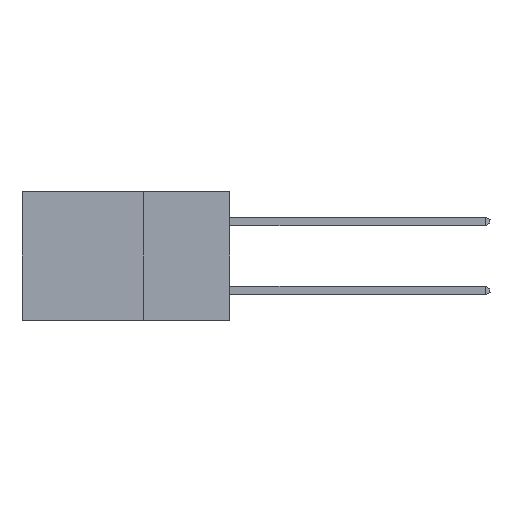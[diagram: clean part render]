
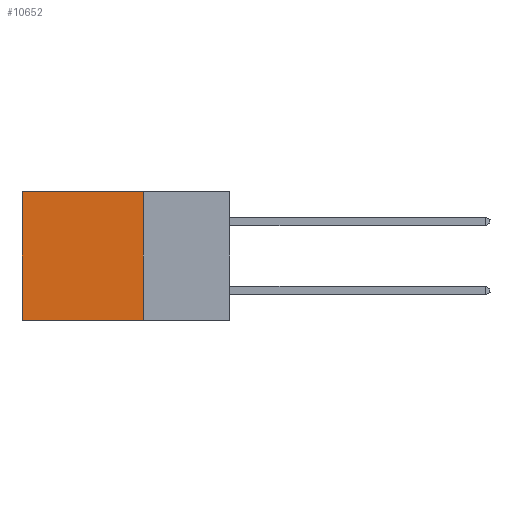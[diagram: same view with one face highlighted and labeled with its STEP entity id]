
A CAD part, left-side view. The second image highlights one B-rep face of the part: STEP entity #10652.
In plain terms, the highlighted planar face has unit normal (-1, 0, 0).
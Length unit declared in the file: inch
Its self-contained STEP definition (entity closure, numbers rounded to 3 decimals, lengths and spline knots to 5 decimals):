
#210 = VERTEX_POINT ( 'NONE', #7712 ) ;
#901 = ORIENTED_EDGE ( 'NONE', *, *, #3947, .F. ) ;
#1298 = DIRECTION ( 'NONE',  ( 1., 0., 0. ) ) ;
#1379 = DIRECTION ( 'NONE',  ( 0., 0., -1. ) ) ;
#1572 = CARTESIAN_POINT ( 'NONE',  ( 0.298, 0.25, -0.37 ) ) ;
#2370 = EDGE_CURVE ( 'NONE', #5544, #8849, #4086, .T. ) ;
#2432 = EDGE_LOOP ( 'NONE', ( #6228, #9332, #901, #4699 ) ) ;
#2742 = EDGE_CURVE ( 'NONE', #4283, #210, #8134, .T. ) ;
#3030 = CARTESIAN_POINT ( 'NONE',  ( 0.298, 0.25, -0.37 ) ) ;
#3839 = DIRECTION ( 'NONE',  ( 0., 1., 0. ) ) ;
#3947 = EDGE_CURVE ( 'NONE', #4283, #5544, #10007, .T. ) ;
#4086 = LINE ( 'NONE', #3030, #6116 ) ;
#4283 = VERTEX_POINT ( 'NONE', #8377 ) ;
#4374 = CARTESIAN_POINT ( 'NONE',  ( 0.298, 0.25, 0. ) ) ;
#4481 = CARTESIAN_POINT ( 'NONE',  ( 0.298, 0.25, 0. ) ) ;
#4699 = ORIENTED_EDGE ( 'NONE', *, *, #2742, .T. ) ;
#5544 = VERTEX_POINT ( 'NONE', #1572 ) ;
#5936 = AXIS2_PLACEMENT_3D ( 'NONE', #4481, #1298, #1379 ) ;
#5995 = PLANE ( 'NONE',  #5936 ) ;
#6116 = VECTOR ( 'NONE', #6417, 39.37008 ) ;
#6228 = ORIENTED_EDGE ( 'NONE', *, *, #11028, .T. ) ;
#6417 = DIRECTION ( 'NONE',  ( 0., 1., 0. ) ) ;
#6956 = DIRECTION ( 'NONE',  ( 0., 0., -1. ) ) ;
#7054 = LINE ( 'NONE', #9370, #7986 ) ;
#7712 = CARTESIAN_POINT ( 'NONE',  ( 0.298, 0.6, 0. ) ) ;
#7986 = VECTOR ( 'NONE', #9255, 39.37008 ) ;
#8134 = LINE ( 'NONE', #10534, #8498 ) ;
#8377 = CARTESIAN_POINT ( 'NONE',  ( 0.298, 0.25, 0. ) ) ;
#8498 = VECTOR ( 'NONE', #3839, 39.37008 ) ;
#8849 = VERTEX_POINT ( 'NONE', #10431 ) ;
#9211 = VECTOR ( 'NONE', #6956, 39.37008 ) ;
#9255 = DIRECTION ( 'NONE',  ( 0., 0., -1. ) ) ;
#9332 = ORIENTED_EDGE ( 'NONE', *, *, #2370, .F. ) ;
#9370 = CARTESIAN_POINT ( 'NONE',  ( 0.298, 0.6, 0. ) ) ;
#9551 = FACE_OUTER_BOUND ( 'NONE', #2432, .T. ) ;
#10007 = LINE ( 'NONE', #4374, #9211 ) ;
#10431 = CARTESIAN_POINT ( 'NONE',  ( 0.298, 0.6, -0.37 ) ) ;
#10534 = CARTESIAN_POINT ( 'NONE',  ( 0.298, 0.25, 0. ) ) ;
#10652 = ADVANCED_FACE ( 'NONE', ( #9551 ), #5995, .F. ) ;
#11028 = EDGE_CURVE ( 'NONE', #210, #8849, #7054, .T. ) ;
